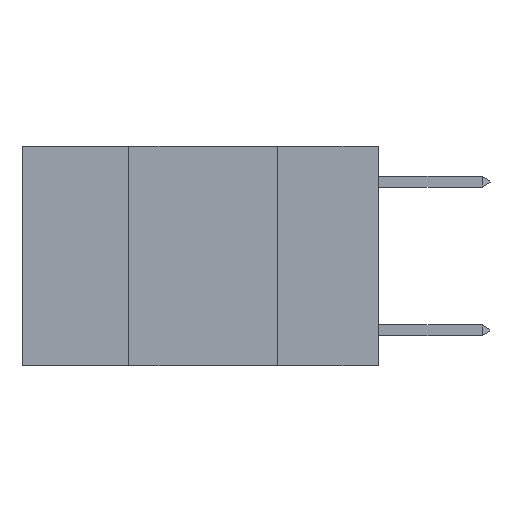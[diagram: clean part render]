
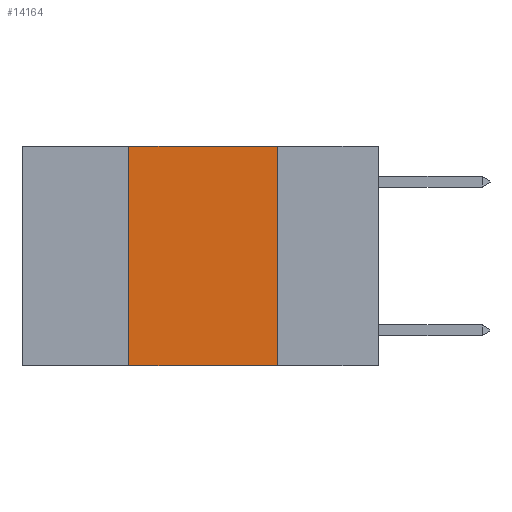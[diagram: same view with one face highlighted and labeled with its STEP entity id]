
A CAD part, left-side view. The second image highlights one B-rep face of the part: STEP entity #14164.
In plain terms, the highlighted planar face has unit normal (-1, 0, 0).
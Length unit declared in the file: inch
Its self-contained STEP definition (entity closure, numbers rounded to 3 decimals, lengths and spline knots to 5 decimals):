
#1056 = CARTESIAN_POINT ( 'NONE',  ( 0., 0.6, 0. ) ) ;
#1092 = AXIS2_PLACEMENT_3D ( 'NONE', #17214, #18977, #8146 ) ;
#2355 = FACE_OUTER_BOUND ( 'NONE', #4680, .T. ) ;
#2808 = VERTEX_POINT ( 'NONE', #17320 ) ;
#3134 = LINE ( 'NONE', #7998, #7356 ) ;
#4532 = PLANE ( 'NONE',  #1092 ) ;
#4680 = EDGE_LOOP ( 'NONE', ( #11348, #11486, #11575, #11724 ) ) ;
#4748 = VECTOR ( 'NONE', #8484, 39.37008 ) ;
#7356 = VECTOR ( 'NONE', #9713, 39.37008 ) ;
#7998 = CARTESIAN_POINT ( 'NONE',  ( 0., 0.17, 0. ) ) ;
#8104 = LINE ( 'NONE', #1056, #17209 ) ;
#8146 = DIRECTION ( 'NONE',  ( 0., 0., -1. ) ) ;
#8484 = DIRECTION ( 'NONE',  ( 0., -1., 0. ) ) ;
#8811 = EDGE_CURVE ( 'NONE', #2808, #19197, #3134, .T. ) ;
#9713 = DIRECTION ( 'NONE',  ( 0., 0., -1. ) ) ;
#10066 = EDGE_CURVE ( 'NONE', #14513, #19197, #14947, .T. ) ;
#11348 = ORIENTED_EDGE ( 'NONE', *, *, #8811, .F. ) ;
#11486 = ORIENTED_EDGE ( 'NONE', *, *, #18781, .F. ) ;
#11575 = ORIENTED_EDGE ( 'NONE', *, *, #11748, .F. ) ;
#11724 = ORIENTED_EDGE ( 'NONE', *, *, #10066, .T. ) ;
#11748 = EDGE_CURVE ( 'NONE', #14513, #14455, #22193, .T. ) ;
#11874 = DIRECTION ( 'NONE',  ( 0., -1., 0. ) ) ;
#12105 = CARTESIAN_POINT ( 'NONE',  ( 0., 0.6, -0.37 ) ) ;
#13783 = VECTOR ( 'NONE', #20321, 39.37008 ) ;
#14164 = ADVANCED_FACE ( 'NONE', ( #2355 ), #4532, .F. ) ;
#14319 = CARTESIAN_POINT ( 'NONE',  ( 0., 0.17, -0.37 ) ) ;
#14455 = VERTEX_POINT ( 'NONE', #19679 ) ;
#14490 = CARTESIAN_POINT ( 'NONE',  ( 0., 0.42, -0.37 ) ) ;
#14513 = VERTEX_POINT ( 'NONE', #14490 ) ;
#14947 = LINE ( 'NONE', #12105, #4748 ) ;
#17209 = VECTOR ( 'NONE', #11874, 39.37008 ) ;
#17214 = CARTESIAN_POINT ( 'NONE',  ( 0., 0.6, 0. ) ) ;
#17320 = CARTESIAN_POINT ( 'NONE',  ( 0., 0.17, 0. ) ) ;
#18544 = CARTESIAN_POINT ( 'NONE',  ( 0., 0.42, 0. ) ) ;
#18781 = EDGE_CURVE ( 'NONE', #14455, #2808, #8104, .T. ) ;
#18977 = DIRECTION ( 'NONE',  ( 1., 0., 0. ) ) ;
#19197 = VERTEX_POINT ( 'NONE', #14319 ) ;
#19679 = CARTESIAN_POINT ( 'NONE',  ( 0., 0.42, 0. ) ) ;
#20321 = DIRECTION ( 'NONE',  ( 0., 0., 1. ) ) ;
#22193 = LINE ( 'NONE', #18544, #13783 ) ;
